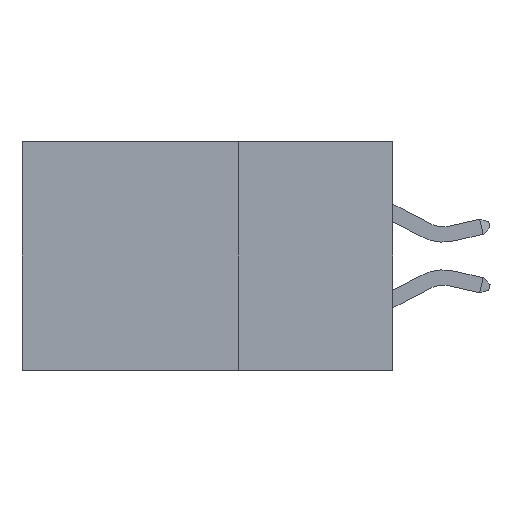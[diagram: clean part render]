
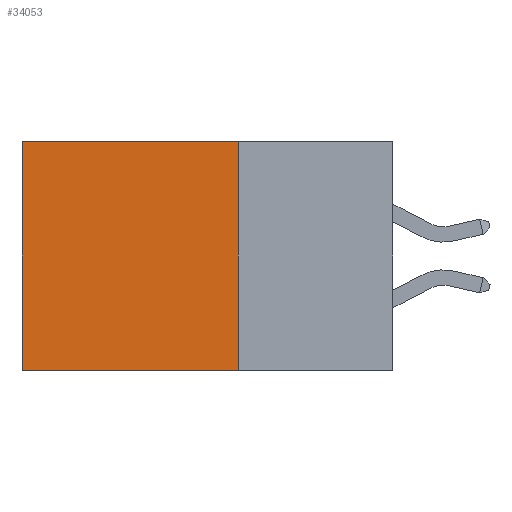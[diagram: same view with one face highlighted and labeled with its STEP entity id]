
A CAD part, left-side view. The second image highlights one B-rep face of the part: STEP entity #34053.
In plain terms, the highlighted planar face has unit normal (-1, 0, 0).
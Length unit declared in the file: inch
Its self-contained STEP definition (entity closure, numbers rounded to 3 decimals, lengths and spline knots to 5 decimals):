
#5718 = LINE ( 'NONE', #22751, #35512 ) ;
#6662 = CARTESIAN_POINT ( 'NONE',  ( 0.2875, 0.6, 0. ) ) ;
#8757 = CARTESIAN_POINT ( 'NONE',  ( 0.2875, 0.6, 0. ) ) ;
#8889 = DIRECTION ( 'NONE',  ( 0., 0., -1. ) ) ;
#8935 = VERTEX_POINT ( 'NONE', #27414 ) ;
#9047 = ORIENTED_EDGE ( 'NONE', *, *, #30874, .F. ) ;
#9166 = LINE ( 'NONE', #28156, #16006 ) ;
#9386 = ORIENTED_EDGE ( 'NONE', *, *, #34093, .T. ) ;
#11096 = ORIENTED_EDGE ( 'NONE', *, *, #39745, .F. ) ;
#11164 = VECTOR ( 'NONE', #8889, 39.37008 ) ;
#11643 = PLANE ( 'NONE',  #34163 ) ;
#11768 = DIRECTION ( 'NONE',  ( 1., 0., 0. ) ) ;
#12239 = LINE ( 'NONE', #33075, #19566 ) ;
#13552 = EDGE_LOOP ( 'NONE', ( #9386, #9047, #11096, #22874 ) ) ;
#14394 = DIRECTION ( 'NONE',  ( 0., 0., -1. ) ) ;
#16006 = VECTOR ( 'NONE', #34309, 39.37008 ) ;
#16629 = CARTESIAN_POINT ( 'NONE',  ( 0.2875, 0.6, -0.37 ) ) ;
#18172 = CARTESIAN_POINT ( 'NONE',  ( 0.2875, 0.25, 0. ) ) ;
#19566 = VECTOR ( 'NONE', #14394, 39.37008 ) ;
#22751 = CARTESIAN_POINT ( 'NONE',  ( 0.2875, 0.25, -0.37 ) ) ;
#22874 = ORIENTED_EDGE ( 'NONE', *, *, #35514, .T. ) ;
#26023 = DIRECTION ( 'NONE',  ( 0., 1., 0. ) ) ;
#26815 = VERTEX_POINT ( 'NONE', #16629 ) ;
#27414 = CARTESIAN_POINT ( 'NONE',  ( 0.2875, 0.25, 0. ) ) ;
#27426 = DIRECTION ( 'NONE',  ( 0., 0., -1. ) ) ;
#27641 = VERTEX_POINT ( 'NONE', #34174 ) ;
#28156 = CARTESIAN_POINT ( 'NONE',  ( 0.2875, 0.25, 0. ) ) ;
#28733 = FACE_OUTER_BOUND ( 'NONE', #13552, .T. ) ;
#30874 = EDGE_CURVE ( 'NONE', #27641, #26815, #5718, .T. ) ;
#33075 = CARTESIAN_POINT ( 'NONE',  ( 0.2875, 0.25, 0. ) ) ;
#34053 = ADVANCED_FACE ( 'NONE', ( #28733 ), #11643, .F. ) ;
#34093 = EDGE_CURVE ( 'NONE', #34974, #26815, #38972, .T. ) ;
#34163 = AXIS2_PLACEMENT_3D ( 'NONE', #18172, #11768, #27426 ) ;
#34174 = CARTESIAN_POINT ( 'NONE',  ( 0.2875, 0.25, -0.37 ) ) ;
#34309 = DIRECTION ( 'NONE',  ( 0., 1., 0. ) ) ;
#34974 = VERTEX_POINT ( 'NONE', #6662 ) ;
#35512 = VECTOR ( 'NONE', #26023, 39.37008 ) ;
#35514 = EDGE_CURVE ( 'NONE', #8935, #34974, #9166, .T. ) ;
#38972 = LINE ( 'NONE', #8757, #11164 ) ;
#39745 = EDGE_CURVE ( 'NONE', #8935, #27641, #12239, .T. ) ;
